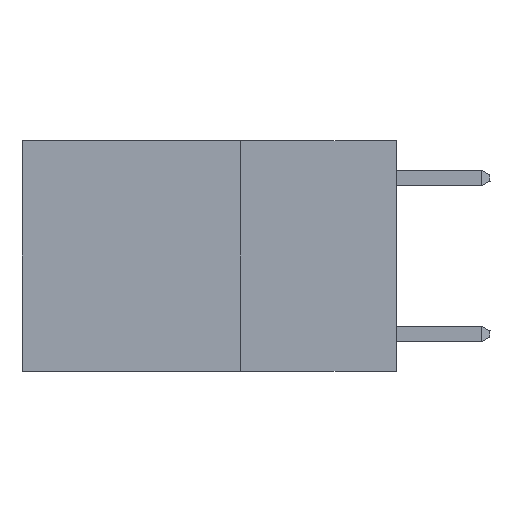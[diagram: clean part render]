
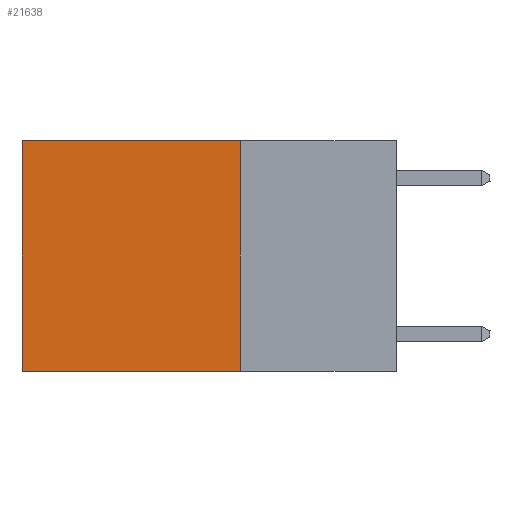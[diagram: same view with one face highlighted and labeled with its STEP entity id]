
A CAD part, left-side view. The second image highlights one B-rep face of the part: STEP entity #21638.
In plain terms, the highlighted planar face has unit normal (-1, 0, 0).
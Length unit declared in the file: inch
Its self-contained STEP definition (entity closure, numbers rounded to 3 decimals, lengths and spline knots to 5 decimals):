
#2244 = CARTESIAN_POINT ( 'NONE',  ( 0.2625, 0.25, -0.37 ) ) ;
#2491 = VECTOR ( 'NONE', #29716, 39.37008 ) ;
#2519 = VERTEX_POINT ( 'NONE', #3598 ) ;
#3039 = LINE ( 'NONE', #18988, #20937 ) ;
#3598 = CARTESIAN_POINT ( 'NONE',  ( 0.2625, 0.6, 0. ) ) ;
#4254 = DIRECTION ( 'NONE',  ( 1., 0., 0. ) ) ;
#5045 = ORIENTED_EDGE ( 'NONE', *, *, #23096, .T. ) ;
#5671 = DIRECTION ( 'NONE',  ( 0., 1., 0. ) ) ;
#7189 = CARTESIAN_POINT ( 'NONE',  ( 0.2625, 0.25, 0. ) ) ;
#9058 = ORIENTED_EDGE ( 'NONE', *, *, #12403, .T. ) ;
#9297 = DIRECTION ( 'NONE',  ( 0., 0., -1. ) ) ;
#12403 = EDGE_CURVE ( 'NONE', #20426, #2519, #24323, .T. ) ;
#14052 = VECTOR ( 'NONE', #9297, 39.37008 ) ;
#14189 = ORIENTED_EDGE ( 'NONE', *, *, #26246, .F. ) ;
#14371 = ORIENTED_EDGE ( 'NONE', *, *, #25416, .F. ) ;
#14764 = CARTESIAN_POINT ( 'NONE',  ( 0.2625, 0.25, 0. ) ) ;
#15670 = CARTESIAN_POINT ( 'NONE',  ( 0.2625, 0.6, -0.37 ) ) ;
#15933 = FACE_OUTER_BOUND ( 'NONE', #28836, .T. ) ;
#17601 = DIRECTION ( 'NONE',  ( 0., 0., -1. ) ) ;
#18332 = LINE ( 'NONE', #27608, #2491 ) ;
#18988 = CARTESIAN_POINT ( 'NONE',  ( 0.2625, 0.25, -0.37 ) ) ;
#20426 = VERTEX_POINT ( 'NONE', #7189 ) ;
#20937 = VECTOR ( 'NONE', #21566, 39.37008 ) ;
#21458 = VERTEX_POINT ( 'NONE', #2244 ) ;
#21566 = DIRECTION ( 'NONE',  ( 0., 1., 0. ) ) ;
#21638 = ADVANCED_FACE ( 'NONE', ( #15933 ), #29287, .F. ) ;
#23096 = EDGE_CURVE ( 'NONE', #2519, #27759, #23255, .T. ) ;
#23103 = CARTESIAN_POINT ( 'NONE',  ( 0.2625, 0.6, 0. ) ) ;
#23255 = LINE ( 'NONE', #23103, #14052 ) ;
#24323 = LINE ( 'NONE', #14764, #29198 ) ;
#25046 = CARTESIAN_POINT ( 'NONE',  ( 0.2625, 0.25, 0. ) ) ;
#25416 = EDGE_CURVE ( 'NONE', #20426, #21458, #18332, .T. ) ;
#26246 = EDGE_CURVE ( 'NONE', #21458, #27759, #3039, .T. ) ;
#27608 = CARTESIAN_POINT ( 'NONE',  ( 0.2625, 0.25, 0. ) ) ;
#27759 = VERTEX_POINT ( 'NONE', #15670 ) ;
#28836 = EDGE_LOOP ( 'NONE', ( #5045, #14189, #14371, #9058 ) ) ;
#29198 = VECTOR ( 'NONE', #5671, 39.37008 ) ;
#29287 = PLANE ( 'NONE',  #29471 ) ;
#29471 = AXIS2_PLACEMENT_3D ( 'NONE', #25046, #4254, #17601 ) ;
#29716 = DIRECTION ( 'NONE',  ( 0., 0., -1. ) ) ;
